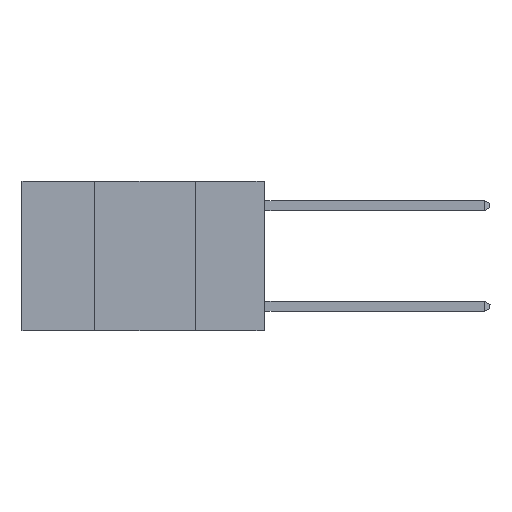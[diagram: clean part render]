
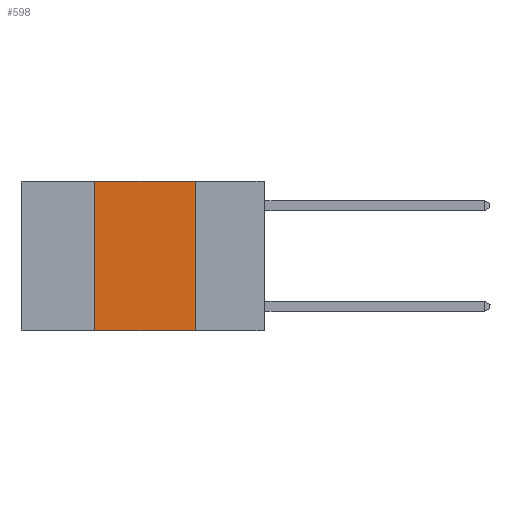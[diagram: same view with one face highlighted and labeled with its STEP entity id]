
A CAD part, left-side view. The second image highlights one B-rep face of the part: STEP entity #598.
In plain terms, the highlighted planar face has unit normal (-1, 0, 0).
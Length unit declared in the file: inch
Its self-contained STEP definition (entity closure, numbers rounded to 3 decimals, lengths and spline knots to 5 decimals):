
#598 = ADVANCED_FACE ( 'NONE', ( #5893 ), #7251, .F. ) ;
#637 = ORIENTED_EDGE ( 'NONE', *, *, #10954, .F. ) ;
#668 = CARTESIAN_POINT ( 'NONE',  ( 0., 0.42, -0.37 ) ) ;
#1137 = EDGE_CURVE ( 'NONE', #7977, #10750, #2835, .T. ) ;
#1517 = DIRECTION ( 'NONE',  ( 0., 0., -1. ) ) ;
#1669 = VECTOR ( 'NONE', #4668, 39.37008 ) ;
#1794 = CARTESIAN_POINT ( 'NONE',  ( 0., 0.6, -0.37 ) ) ;
#1906 = VERTEX_POINT ( 'NONE', #668 ) ;
#2105 = LINE ( 'NONE', #7005, #2387 ) ;
#2387 = VECTOR ( 'NONE', #1517, 39.37008 ) ;
#2436 = VERTEX_POINT ( 'NONE', #10662 ) ;
#2835 = LINE ( 'NONE', #4284, #9713 ) ;
#3526 = CARTESIAN_POINT ( 'NONE',  ( 0., 0.17, 0. ) ) ;
#3913 = VECTOR ( 'NONE', #9089, 39.37008 ) ;
#4270 = DIRECTION ( 'NONE',  ( 0., -1., 0. ) ) ;
#4284 = CARTESIAN_POINT ( 'NONE',  ( 0., 0.6, 0. ) ) ;
#4668 = DIRECTION ( 'NONE',  ( 0., -1., 0. ) ) ;
#4704 = CARTESIAN_POINT ( 'NONE',  ( 0., 0.42, 0. ) ) ;
#4784 = LINE ( 'NONE', #1794, #1669 ) ;
#5282 = ORIENTED_EDGE ( 'NONE', *, *, #10683, .F. ) ;
#5893 = FACE_OUTER_BOUND ( 'NONE', #7359, .T. ) ;
#7005 = CARTESIAN_POINT ( 'NONE',  ( 0., 0.17, 0. ) ) ;
#7232 = DIRECTION ( 'NONE',  ( 0., 0., -1. ) ) ;
#7240 = DIRECTION ( 'NONE',  ( 1., 0., 0. ) ) ;
#7251 = PLANE ( 'NONE',  #10012 ) ;
#7301 = CARTESIAN_POINT ( 'NONE',  ( 0., 0.6, 0. ) ) ;
#7359 = EDGE_LOOP ( 'NONE', ( #5282, #7591, #637, #7874 ) ) ;
#7591 = ORIENTED_EDGE ( 'NONE', *, *, #1137, .F. ) ;
#7874 = ORIENTED_EDGE ( 'NONE', *, *, #10931, .T. ) ;
#7977 = VERTEX_POINT ( 'NONE', #8427 ) ;
#8427 = CARTESIAN_POINT ( 'NONE',  ( 0., 0.42, 0. ) ) ;
#9089 = DIRECTION ( 'NONE',  ( 0., 0., 1. ) ) ;
#9713 = VECTOR ( 'NONE', #4270, 39.37008 ) ;
#10012 = AXIS2_PLACEMENT_3D ( 'NONE', #7301, #7240, #7232 ) ;
#10662 = CARTESIAN_POINT ( 'NONE',  ( 0., 0.17, -0.37 ) ) ;
#10683 = EDGE_CURVE ( 'NONE', #10750, #2436, #2105, .T. ) ;
#10750 = VERTEX_POINT ( 'NONE', #3526 ) ;
#10873 = LINE ( 'NONE', #4704, #3913 ) ;
#10931 = EDGE_CURVE ( 'NONE', #1906, #2436, #4784, .T. ) ;
#10954 = EDGE_CURVE ( 'NONE', #1906, #7977, #10873, .T. ) ;
